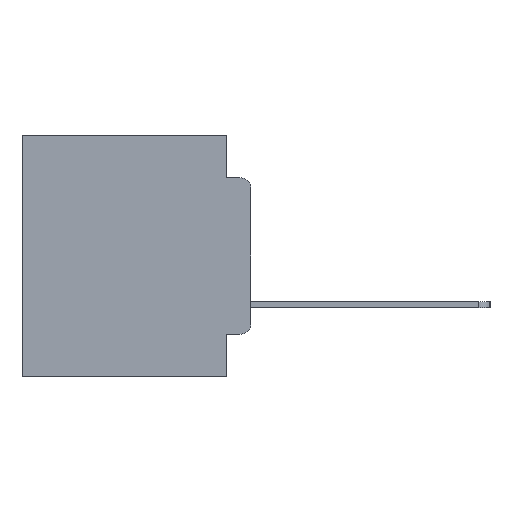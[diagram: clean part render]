
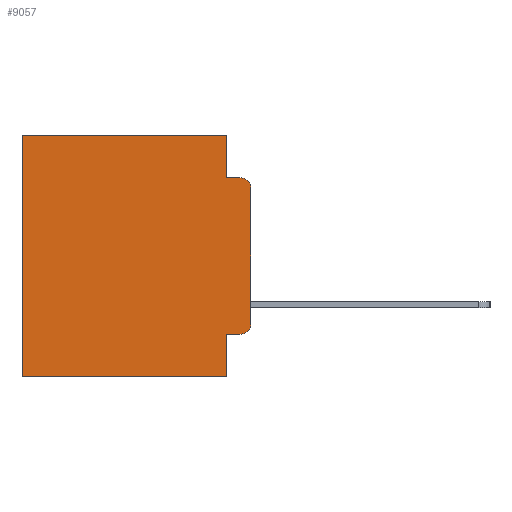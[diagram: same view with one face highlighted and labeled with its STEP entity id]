
A CAD part, left-side view. The second image highlights one B-rep face of the part: STEP entity #9057.
In plain terms, the highlighted planar face has unit normal (-1, 0, 0).
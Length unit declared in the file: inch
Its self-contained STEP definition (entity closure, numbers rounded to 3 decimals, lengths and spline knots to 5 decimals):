
#947 = VERTEX_POINT ( 'NONE', #1158 ) ;
#1058 = ORIENTED_EDGE ( 'NONE', *, *, #10976, .T. ) ;
#1158 = CARTESIAN_POINT ( 'NONE',  ( 0.298, 0.473, -0.5 ) ) ;
#1766 = DIRECTION ( 'NONE',  ( 0., 0., -1. ) ) ;
#2106 = VERTEX_POINT ( 'NONE', #26121 ) ;
#2128 = VERTEX_POINT ( 'NONE', #18148 ) ;
#2652 = LINE ( 'NONE', #5735, #18684 ) ;
#2869 = CIRCLE ( 'NONE', #18825, 0.02 ) ;
#3106 = ORIENTED_EDGE ( 'NONE', *, *, #8491, .T. ) ;
#3427 = ORIENTED_EDGE ( 'NONE', *, *, #8523, .F. ) ;
#3437 = AXIS2_PLACEMENT_3D ( 'NONE', #12335, #25717, #14338 ) ;
#3547 = VECTOR ( 'NONE', #20484, 39.37008 ) ;
#4238 = LINE ( 'NONE', #14518, #14814 ) ;
#4795 = ORIENTED_EDGE ( 'NONE', *, *, #8493, .F. ) ;
#5090 = VERTEX_POINT ( 'NONE', #5937 ) ;
#5735 = CARTESIAN_POINT ( 'NONE',  ( 0.298, 0., 0. ) ) ;
#5937 = CARTESIAN_POINT ( 'NONE',  ( 0.298, 0.051, -0.4115 ) ) ;
#6230 = CARTESIAN_POINT ( 'NONE',  ( 0.298, 0.051, -0.0885 ) ) ;
#6272 = CIRCLE ( 'NONE', #3437, 0.02 ) ;
#7932 = VERTEX_POINT ( 'NONE', #15074 ) ;
#8088 = CARTESIAN_POINT ( 'NONE',  ( 0.298, 0.051, -0.4115 ) ) ;
#8452 = EDGE_CURVE ( 'NONE', #10445, #9839, #6272, .T. ) ;
#8461 = EDGE_CURVE ( 'NONE', #5090, #10445, #16714, .T. ) ;
#8490 = EDGE_CURVE ( 'NONE', #5090, #2106, #9997, .T. ) ;
#8491 = EDGE_CURVE ( 'NONE', #12239, #947, #4238, .T. ) ;
#8493 = EDGE_CURVE ( 'NONE', #12225, #2128, #20071, .T. ) ;
#8523 = EDGE_CURVE ( 'NONE', #2128, #12998, #14167, .T. ) ;
#8531 = EDGE_CURVE ( 'NONE', #7932, #12998, #2869, .T. ) ;
#8537 = DIRECTION ( 'NONE',  ( -1., 0., 0. ) ) ;
#8562 = EDGE_CURVE ( 'NONE', #7932, #9839, #18271, .T. ) ;
#8960 = DIRECTION ( 'NONE',  ( 0., 0., -1. ) ) ;
#9057 = ADVANCED_FACE ( 'NONE', ( #20620 ), #19085, .F. ) ;
#9112 = EDGE_CURVE ( 'NONE', #2106, #947, #23179, .T. ) ;
#9243 = ORIENTED_EDGE ( 'NONE', *, *, #8461, .T. ) ;
#9839 = VERTEX_POINT ( 'NONE', #18785 ) ;
#9997 = LINE ( 'NONE', #25879, #24923 ) ;
#10445 = VERTEX_POINT ( 'NONE', #17786 ) ;
#10976 = EDGE_CURVE ( 'NONE', #12225, #12239, #2652, .T. ) ;
#12225 = VERTEX_POINT ( 'NONE', #25177 ) ;
#12239 = VERTEX_POINT ( 'NONE', #23207 ) ;
#12335 = CARTESIAN_POINT ( 'NONE',  ( 0.298, 0.02, -0.3915 ) ) ;
#12504 = DIRECTION ( 'NONE',  ( 0., 0., -1. ) ) ;
#12846 = CARTESIAN_POINT ( 'NONE',  ( 0.298, 0., 0. ) ) ;
#12878 = VECTOR ( 'NONE', #21256, 39.37008 ) ;
#12998 = VERTEX_POINT ( 'NONE', #24733 ) ;
#14058 = ORIENTED_EDGE ( 'NONE', *, *, #8562, .F. ) ;
#14167 = LINE ( 'NONE', #6230, #23815 ) ;
#14338 = DIRECTION ( 'NONE',  ( 0., 0., -1. ) ) ;
#14518 = CARTESIAN_POINT ( 'NONE',  ( 0.298, 0.473, 0. ) ) ;
#14697 = DIRECTION ( 'NONE',  ( 0., -1., 0. ) ) ;
#14814 = VECTOR ( 'NONE', #1766, 39.37008 ) ;
#15074 = CARTESIAN_POINT ( 'NONE',  ( 0.298, 0., -0.1085 ) ) ;
#15361 = ORIENTED_EDGE ( 'NONE', *, *, #8452, .T. ) ;
#16083 = VECTOR ( 'NONE', #16389, 39.37008 ) ;
#16276 = DIRECTION ( 'NONE',  ( 0., 1., 0. ) ) ;
#16389 = DIRECTION ( 'NONE',  ( 0., -1., 0. ) ) ;
#16714 = LINE ( 'NONE', #8088, #16083 ) ;
#17786 = CARTESIAN_POINT ( 'NONE',  ( 0.298, 0.02, -0.4115 ) ) ;
#18148 = CARTESIAN_POINT ( 'NONE',  ( 0.298, 0.051, -0.0885 ) ) ;
#18271 = LINE ( 'NONE', #12846, #22662 ) ;
#18543 = CARTESIAN_POINT ( 'NONE',  ( 0.298, 0.051, 0. ) ) ;
#18684 = VECTOR ( 'NONE', #16276, 39.37008 ) ;
#18785 = CARTESIAN_POINT ( 'NONE',  ( 0.298, 0., -0.3915 ) ) ;
#18798 = ORIENTED_EDGE ( 'NONE', *, *, #8490, .F. ) ;
#18825 = AXIS2_PLACEMENT_3D ( 'NONE', #20633, #8537, #22483 ) ;
#19056 = EDGE_LOOP ( 'NONE', ( #14058, #19378, #3427, #4795, #1058, #3106, #25699, #18798, #9243, #15361 ) ) ;
#19085 = PLANE ( 'NONE',  #26066 ) ;
#19352 = CARTESIAN_POINT ( 'NONE',  ( 0.298, 0., -0.5 ) ) ;
#19378 = ORIENTED_EDGE ( 'NONE', *, *, #8531, .T. ) ;
#20071 = LINE ( 'NONE', #18543, #3547 ) ;
#20484 = DIRECTION ( 'NONE',  ( 0., 0., -1. ) ) ;
#20620 = FACE_OUTER_BOUND ( 'NONE', #19056, .T. ) ;
#20633 = CARTESIAN_POINT ( 'NONE',  ( 0.298, 0.02, -0.1085 ) ) ;
#21013 = DIRECTION ( 'NONE',  ( 1., 0., 0. ) ) ;
#21256 = DIRECTION ( 'NONE',  ( 0., 1., 0. ) ) ;
#22483 = DIRECTION ( 'NONE',  ( 0., 0., -1. ) ) ;
#22662 = VECTOR ( 'NONE', #24371, 39.37008 ) ;
#23179 = LINE ( 'NONE', #19352, #12878 ) ;
#23207 = CARTESIAN_POINT ( 'NONE',  ( 0.298, 0.473, 0. ) ) ;
#23815 = VECTOR ( 'NONE', #14697, 39.37008 ) ;
#24371 = DIRECTION ( 'NONE',  ( 0., 0., -1. ) ) ;
#24568 = CARTESIAN_POINT ( 'NONE',  ( 0.298, 0., 0. ) ) ;
#24733 = CARTESIAN_POINT ( 'NONE',  ( 0.298, 0.02, -0.0885 ) ) ;
#24923 = VECTOR ( 'NONE', #12504, 39.37008 ) ;
#25177 = CARTESIAN_POINT ( 'NONE',  ( 0.298, 0.051, 0. ) ) ;
#25699 = ORIENTED_EDGE ( 'NONE', *, *, #9112, .F. ) ;
#25717 = DIRECTION ( 'NONE',  ( -1., 0., 0. ) ) ;
#25879 = CARTESIAN_POINT ( 'NONE',  ( 0.298, 0.051, 0. ) ) ;
#26066 = AXIS2_PLACEMENT_3D ( 'NONE', #24568, #21013, #8960 ) ;
#26121 = CARTESIAN_POINT ( 'NONE',  ( 0.298, 0.051, -0.5 ) ) ;
